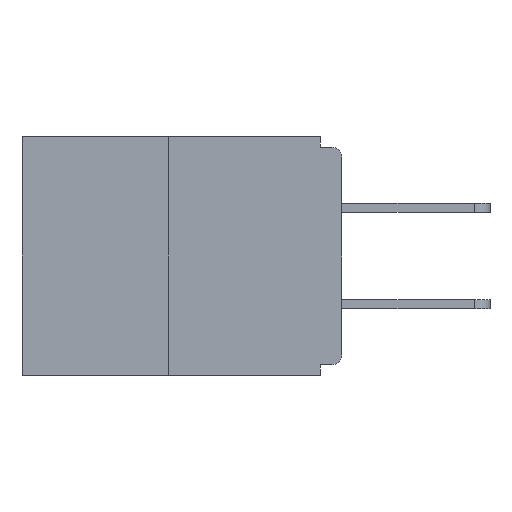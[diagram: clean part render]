
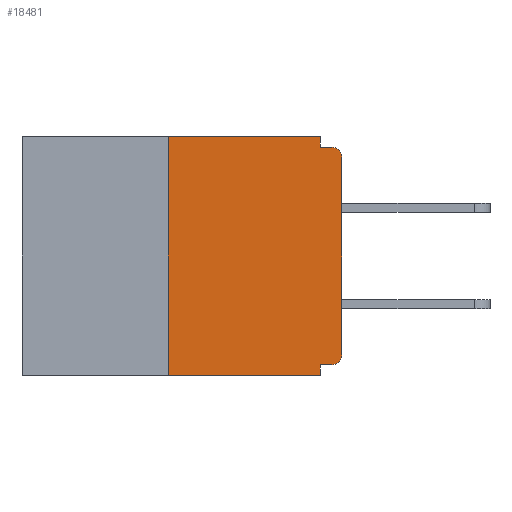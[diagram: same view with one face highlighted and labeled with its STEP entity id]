
A CAD part, left-side view. The second image highlights one B-rep face of the part: STEP entity #18481.
In plain terms, the highlighted planar face has unit normal (-1, 0, 0).
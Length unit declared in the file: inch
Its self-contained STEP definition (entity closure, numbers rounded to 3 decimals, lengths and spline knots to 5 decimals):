
#23 = CARTESIAN_POINT ( 'NONE',  ( 0., 0.031, -0.343 ) ) ;
#217 = VERTEX_POINT ( 'NONE', #12166 ) ;
#276 = LINE ( 'NONE', #9148, #16510 ) ;
#417 = CARTESIAN_POINT ( 'NONE',  ( 0., 0.031, 0. ) ) ;
#561 = VERTEX_POINT ( 'NONE', #14937 ) ;
#781 = CARTESIAN_POINT ( 'NONE',  ( 0., 0.031, -0.015 ) ) ;
#848 = DIRECTION ( 'NONE',  ( 0., 0., -1. ) ) ;
#1705 = AXIS2_PLACEMENT_3D ( 'NONE', #18175, #9965, #8089 ) ;
#1802 = VERTEX_POINT ( 'NONE', #16092 ) ;
#2154 = ORIENTED_EDGE ( 'NONE', *, *, #10433, .F. ) ;
#2465 = DIRECTION ( 'NONE',  ( 0., 0., 1. ) ) ;
#2610 = ORIENTED_EDGE ( 'NONE', *, *, #20170, .T. ) ;
#2891 = CARTESIAN_POINT ( 'NONE',  ( 0., 0.031, -0.328 ) ) ;
#3126 = CIRCLE ( 'NONE', #19551, 0.015 ) ;
#3449 = FACE_OUTER_BOUND ( 'NONE', #6446, .T. ) ;
#4559 = VECTOR ( 'NONE', #18933, 39.37008 ) ;
#4569 = CARTESIAN_POINT ( 'NONE',  ( 0., 0.031, 0. ) ) ;
#4943 = EDGE_CURVE ( 'NONE', #12420, #6617, #18186, .T. ) ;
#5096 = EDGE_CURVE ( 'NONE', #6617, #12789, #16857, .T. ) ;
#5231 = EDGE_CURVE ( 'NONE', #561, #1802, #15492, .T. ) ;
#5808 = VECTOR ( 'NONE', #9376, 39.37008 ) ;
#5998 = DIRECTION ( 'NONE',  ( -1., 0., 0. ) ) ;
#6446 = EDGE_LOOP ( 'NONE', ( #2154, #14304, #16540, #14161, #16996, #2610, #17213, #7891, #12579, #20333 ) ) ;
#6617 = VERTEX_POINT ( 'NONE', #781 ) ;
#6999 = CARTESIAN_POINT ( 'NONE',  ( 0., 0., -0.313 ) ) ;
#7281 = DIRECTION ( 'NONE',  ( 0., 0., -1. ) ) ;
#7389 = CARTESIAN_POINT ( 'NONE',  ( 0., 0.46, -0.343 ) ) ;
#7891 = ORIENTED_EDGE ( 'NONE', *, *, #14948, .T. ) ;
#8089 = DIRECTION ( 'NONE',  ( 0., 0., -1. ) ) ;
#8802 = CARTESIAN_POINT ( 'NONE',  ( 0., 0.015, -0.03 ) ) ;
#9011 = CARTESIAN_POINT ( 'NONE',  ( 0., 0., 0. ) ) ;
#9111 = CARTESIAN_POINT ( 'NONE',  ( 0., 0., -0.015 ) ) ;
#9148 = CARTESIAN_POINT ( 'NONE',  ( 0., 0.031, -0.343 ) ) ;
#9214 = LINE ( 'NONE', #18810, #16300 ) ;
#9376 = DIRECTION ( 'NONE',  ( 0., -1., 0. ) ) ;
#9527 = CARTESIAN_POINT ( 'NONE',  ( 0., 0.015, -0.328 ) ) ;
#9554 = EDGE_CURVE ( 'NONE', #21697, #14761, #9214, .T. ) ;
#9965 = DIRECTION ( 'NONE',  ( 1., 0., 0. ) ) ;
#10433 = EDGE_CURVE ( 'NONE', #1802, #12420, #13623, .T. ) ;
#10952 = DIRECTION ( 'NONE',  ( 0., 0., -1. ) ) ;
#11318 = VERTEX_POINT ( 'NONE', #23 ) ;
#11325 = VECTOR ( 'NONE', #14019, 39.37008 ) ;
#11593 = EDGE_CURVE ( 'NONE', #14854, #217, #14136, .T. ) ;
#11636 = EDGE_CURVE ( 'NONE', #14761, #11318, #276, .T. ) ;
#11987 = VECTOR ( 'NONE', #15737, 39.37008 ) ;
#12166 = CARTESIAN_POINT ( 'NONE',  ( 0., 0., -0.03 ) ) ;
#12296 = VECTOR ( 'NONE', #2465, 39.37008 ) ;
#12342 = LINE ( 'NONE', #7389, #11987 ) ;
#12420 = VERTEX_POINT ( 'NONE', #417 ) ;
#12579 = ORIENTED_EDGE ( 'NONE', *, *, #5096, .F. ) ;
#12789 = VERTEX_POINT ( 'NONE', #17329 ) ;
#13081 = PLANE ( 'NONE',  #1705 ) ;
#13114 = CARTESIAN_POINT ( 'NONE',  ( 0., 0.25, 0. ) ) ;
#13623 = LINE ( 'NONE', #15993, #5808 ) ;
#13746 = CIRCLE ( 'NONE', #16642, 0.015 ) ;
#14019 = DIRECTION ( 'NONE',  ( 0., -1., 0. ) ) ;
#14136 = LINE ( 'NONE', #9011, #12296 ) ;
#14146 = DIRECTION ( 'NONE',  ( 0., 1., 0. ) ) ;
#14161 = ORIENTED_EDGE ( 'NONE', *, *, #11636, .F. ) ;
#14304 = ORIENTED_EDGE ( 'NONE', *, *, #5231, .F. ) ;
#14761 = VERTEX_POINT ( 'NONE', #2891 ) ;
#14854 = VERTEX_POINT ( 'NONE', #6999 ) ;
#14937 = CARTESIAN_POINT ( 'NONE',  ( 0., 0.25, -0.343 ) ) ;
#14948 = EDGE_CURVE ( 'NONE', #217, #12789, #13746, .T. ) ;
#15492 = LINE ( 'NONE', #13114, #18655 ) ;
#15737 = DIRECTION ( 'NONE',  ( 0., -1., 0. ) ) ;
#15786 = DIRECTION ( 'NONE',  ( -1., 0., 0. ) ) ;
#15993 = CARTESIAN_POINT ( 'NONE',  ( 0., 0.46, 0. ) ) ;
#16092 = CARTESIAN_POINT ( 'NONE',  ( 0., 0.25, 0. ) ) ;
#16300 = VECTOR ( 'NONE', #14146, 39.37008 ) ;
#16510 = VECTOR ( 'NONE', #848, 39.37008 ) ;
#16540 = ORIENTED_EDGE ( 'NONE', *, *, #17643, .T. ) ;
#16642 = AXIS2_PLACEMENT_3D ( 'NONE', #8802, #15786, #7281 ) ;
#16857 = LINE ( 'NONE', #9111, #11325 ) ;
#16996 = ORIENTED_EDGE ( 'NONE', *, *, #9554, .F. ) ;
#17213 = ORIENTED_EDGE ( 'NONE', *, *, #11593, .T. ) ;
#17329 = CARTESIAN_POINT ( 'NONE',  ( 0., 0.015, -0.015 ) ) ;
#17623 = CARTESIAN_POINT ( 'NONE',  ( 0., 0.015, -0.313 ) ) ;
#17643 = EDGE_CURVE ( 'NONE', #561, #11318, #12342, .T. ) ;
#18175 = CARTESIAN_POINT ( 'NONE',  ( 0., 0.46, 0. ) ) ;
#18186 = LINE ( 'NONE', #4569, #4559 ) ;
#18209 = DIRECTION ( 'NONE',  ( 0., 0., 1. ) ) ;
#18481 = ADVANCED_FACE ( 'NONE', ( #3449 ), #13081, .F. ) ;
#18655 = VECTOR ( 'NONE', #18209, 39.37008 ) ;
#18810 = CARTESIAN_POINT ( 'NONE',  ( 0., 0., -0.328 ) ) ;
#18933 = DIRECTION ( 'NONE',  ( 0., 0., -1. ) ) ;
#19551 = AXIS2_PLACEMENT_3D ( 'NONE', #17623, #5998, #10952 ) ;
#20170 = EDGE_CURVE ( 'NONE', #21697, #14854, #3126, .T. ) ;
#20333 = ORIENTED_EDGE ( 'NONE', *, *, #4943, .F. ) ;
#21697 = VERTEX_POINT ( 'NONE', #9527 ) ;
